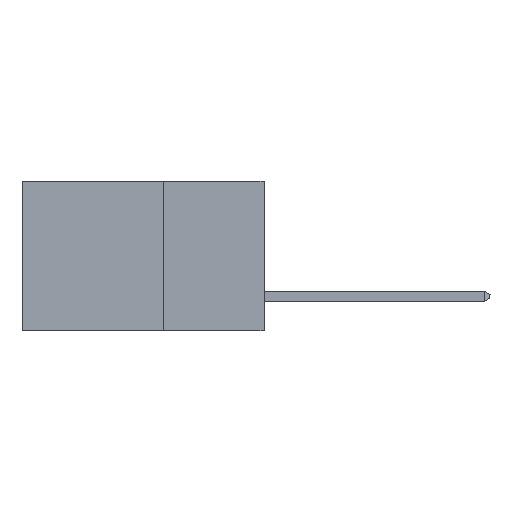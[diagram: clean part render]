
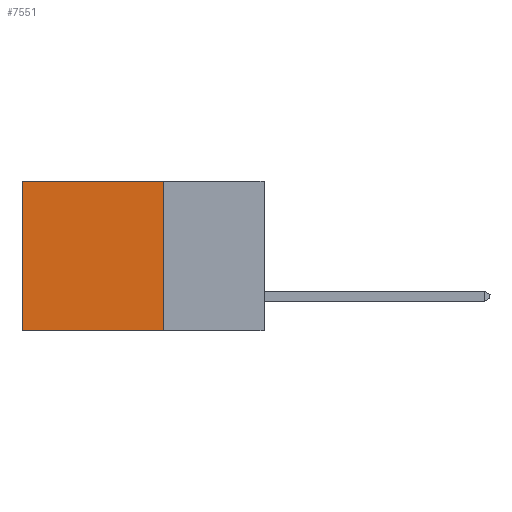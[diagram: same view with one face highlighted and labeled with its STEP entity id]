
A CAD part, left-side view. The second image highlights one B-rep face of the part: STEP entity #7551.
In plain terms, the highlighted planar face has unit normal (-1, 0, 0).
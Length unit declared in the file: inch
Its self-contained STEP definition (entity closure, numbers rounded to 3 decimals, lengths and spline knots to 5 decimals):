
#282 = LINE ( 'NONE', #7922, #4332 ) ;
#545 = LINE ( 'NONE', #2935, #5975 ) ;
#1154 = EDGE_CURVE ( 'NONE', #8994, #12376, #545, .T. ) ;
#1225 = LINE ( 'NONE', #3691, #12687 ) ;
#1728 = EDGE_LOOP ( 'NONE', ( #9293, #14052, #5762, #5606 ) ) ;
#2516 = DIRECTION ( 'NONE',  ( 0., 1., 0. ) ) ;
#2935 = CARTESIAN_POINT ( 'NONE',  ( 0.2615, 0.25, -0.37 ) ) ;
#3219 = VECTOR ( 'NONE', #10861, 39.37008 ) ;
#3552 = VERTEX_POINT ( 'NONE', #6924 ) ;
#3612 = DIRECTION ( 'NONE',  ( 0., 0., -1. ) ) ;
#3691 = CARTESIAN_POINT ( 'NONE',  ( 0.2615, 0.6, -0.37 ) ) ;
#3888 = DIRECTION ( 'NONE',  ( 1., 0., 0. ) ) ;
#4332 = VECTOR ( 'NONE', #2516, 39.37008 ) ;
#4939 = PLANE ( 'NONE',  #11769 ) ;
#5187 = EDGE_CURVE ( 'NONE', #3552, #12376, #1225, .T. ) ;
#5606 = ORIENTED_EDGE ( 'NONE', *, *, #13121, .T. ) ;
#5762 = ORIENTED_EDGE ( 'NONE', *, *, #13450, .F. ) ;
#5975 = VECTOR ( 'NONE', #7280, 39.37008 ) ;
#6142 = CARTESIAN_POINT ( 'NONE',  ( 0.2615, 0.6, -0.37 ) ) ;
#6924 = CARTESIAN_POINT ( 'NONE',  ( 0.2615, 0.6, 0. ) ) ;
#7073 = DIRECTION ( 'NONE',  ( 0., 0., -1. ) ) ;
#7165 = CARTESIAN_POINT ( 'NONE',  ( 0.2615, 0.25, 0. ) ) ;
#7280 = DIRECTION ( 'NONE',  ( 0., 1., 0. ) ) ;
#7551 = ADVANCED_FACE ( 'NONE', ( #12607 ), #4939, .F. ) ;
#7922 = CARTESIAN_POINT ( 'NONE',  ( 0.2615, 0.25, 0. ) ) ;
#8994 = VERTEX_POINT ( 'NONE', #11238 ) ;
#9293 = ORIENTED_EDGE ( 'NONE', *, *, #5187, .T. ) ;
#9776 = CARTESIAN_POINT ( 'NONE',  ( 0.2615, 0.25, -0.37 ) ) ;
#10306 = CARTESIAN_POINT ( 'NONE',  ( 0.2615, 0.25, -0.37 ) ) ;
#10861 = DIRECTION ( 'NONE',  ( 0., 0., -1. ) ) ;
#11238 = CARTESIAN_POINT ( 'NONE',  ( 0.2615, 0.25, -0.37 ) ) ;
#11769 = AXIS2_PLACEMENT_3D ( 'NONE', #10306, #3888, #7073 ) ;
#12376 = VERTEX_POINT ( 'NONE', #6142 ) ;
#12607 = FACE_OUTER_BOUND ( 'NONE', #1728, .T. ) ;
#12687 = VECTOR ( 'NONE', #3612, 39.37008 ) ;
#13121 = EDGE_CURVE ( 'NONE', #14070, #3552, #282, .T. ) ;
#13450 = EDGE_CURVE ( 'NONE', #14070, #8994, #13926, .T. ) ;
#13926 = LINE ( 'NONE', #9776, #3219 ) ;
#14052 = ORIENTED_EDGE ( 'NONE', *, *, #1154, .F. ) ;
#14070 = VERTEX_POINT ( 'NONE', #7165 ) ;
